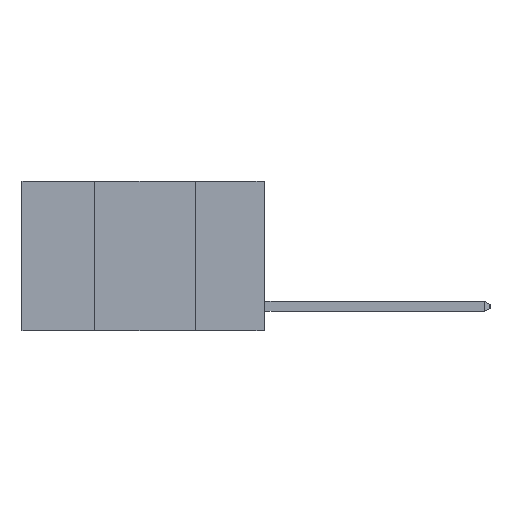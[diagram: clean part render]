
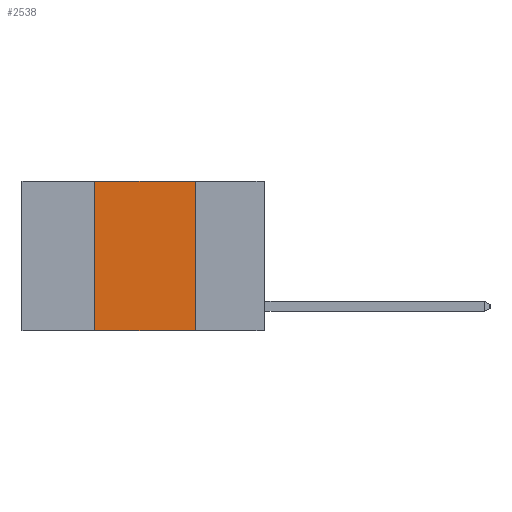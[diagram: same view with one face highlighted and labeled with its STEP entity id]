
A CAD part, left-side view. The second image highlights one B-rep face of the part: STEP entity #2538.
In plain terms, the highlighted planar face has unit normal (-1, 0, 0).
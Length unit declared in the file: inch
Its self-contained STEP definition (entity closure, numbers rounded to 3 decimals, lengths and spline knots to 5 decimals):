
#718 = ORIENTED_EDGE ( 'NONE', *, *, #3737, .F. ) ;
#738 = ORIENTED_EDGE ( 'NONE', *, *, #8081, .F. ) ;
#771 = ORIENTED_EDGE ( 'NONE', *, *, #1659, .F. ) ;
#782 = ORIENTED_EDGE ( 'NONE', *, *, #7115, .T. ) ;
#936 = VERTEX_POINT ( 'NONE', #3671 ) ;
#1145 = CARTESIAN_POINT ( 'NONE',  ( 0., 0.6, 0. ) ) ;
#1154 = LINE ( 'NONE', #1145, #2824 ) ;
#1424 = DIRECTION ( 'NONE',  ( 0., 0., -1. ) ) ;
#1443 = DIRECTION ( 'NONE',  ( 1., 0., 0. ) ) ;
#1559 = CARTESIAN_POINT ( 'NONE',  ( 0., 0.6, 0. ) ) ;
#1631 = PLANE ( 'NONE',  #8235 ) ;
#1659 = EDGE_CURVE ( 'NONE', #936, #6234, #1821, .T. ) ;
#1670 = CARTESIAN_POINT ( 'NONE',  ( 0., 0.42, 0. ) ) ;
#1814 = DIRECTION ( 'NONE',  ( 0., -1., 0. ) ) ;
#1821 = LINE ( 'NONE', #3700, #8127 ) ;
#2320 = CARTESIAN_POINT ( 'NONE',  ( 0., 0.17, -0.37 ) ) ;
#2538 = ADVANCED_FACE ( 'NONE', ( #5324 ), #1631, .F. ) ;
#2607 = VECTOR ( 'NONE', #1814, 39.37008 ) ;
#2824 = VECTOR ( 'NONE', #4494, 39.37008 ) ;
#2846 = LINE ( 'NONE', #3787, #2607 ) ;
#3173 = VECTOR ( 'NONE', #5335, 39.37008 ) ;
#3460 = DIRECTION ( 'NONE',  ( 0., 0., 1. ) ) ;
#3671 = CARTESIAN_POINT ( 'NONE',  ( 0., 0.42, -0.37 ) ) ;
#3700 = CARTESIAN_POINT ( 'NONE',  ( 0., 0.42, 0. ) ) ;
#3737 = EDGE_CURVE ( 'NONE', #4769, #7057, #7750, .T. ) ;
#3787 = CARTESIAN_POINT ( 'NONE',  ( 0., 0.6, -0.37 ) ) ;
#4494 = DIRECTION ( 'NONE',  ( 0., -1., 0. ) ) ;
#4769 = VERTEX_POINT ( 'NONE', #7848 ) ;
#5324 = FACE_OUTER_BOUND ( 'NONE', #6120, .T. ) ;
#5335 = DIRECTION ( 'NONE',  ( 0., 0., -1. ) ) ;
#5949 = CARTESIAN_POINT ( 'NONE',  ( 0., 0.17, 0. ) ) ;
#6120 = EDGE_LOOP ( 'NONE', ( #718, #738, #771, #782 ) ) ;
#6234 = VERTEX_POINT ( 'NONE', #1670 ) ;
#7057 = VERTEX_POINT ( 'NONE', #2320 ) ;
#7115 = EDGE_CURVE ( 'NONE', #936, #7057, #2846, .T. ) ;
#7750 = LINE ( 'NONE', #5949, #3173 ) ;
#7848 = CARTESIAN_POINT ( 'NONE',  ( 0., 0.17, 0. ) ) ;
#8081 = EDGE_CURVE ( 'NONE', #6234, #4769, #1154, .T. ) ;
#8127 = VECTOR ( 'NONE', #3460, 39.37008 ) ;
#8235 = AXIS2_PLACEMENT_3D ( 'NONE', #1559, #1443, #1424 ) ;
